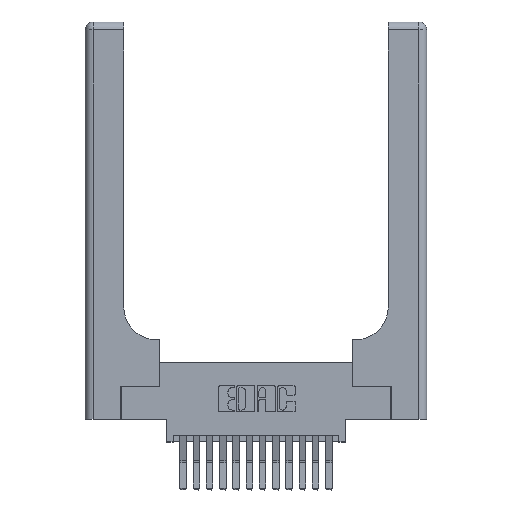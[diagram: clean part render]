
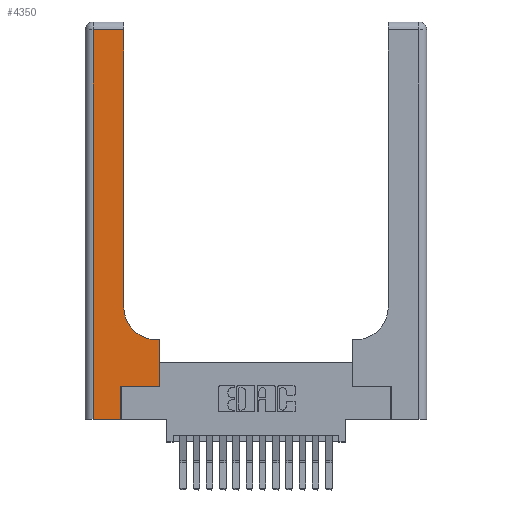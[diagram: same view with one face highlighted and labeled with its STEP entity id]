
A CAD part, top view. The second image highlights one B-rep face of the part: STEP entity #4350.
In plain terms, the highlighted planar face has unit normal (0, 0, 1).
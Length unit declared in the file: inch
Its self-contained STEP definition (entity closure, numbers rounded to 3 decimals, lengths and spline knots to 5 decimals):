
#340 = VERTEX_POINT ( 'NONE', #6474 ) ;
#570 = DIRECTION ( 'NONE',  ( 0., 1., 0. ) ) ;
#598 = CARTESIAN_POINT ( 'NONE',  ( 0.06, 3., 0.37 ) ) ;
#659 = DIRECTION ( 'NONE',  ( 0., 0., -1. ) ) ;
#872 = EDGE_CURVE ( 'NONE', #340, #6453, #12207, .T. ) ;
#1150 = CARTESIAN_POINT ( 'NONE',  ( 0.2915, 2.94, 0.37 ) ) ;
#1258 = VECTOR ( 'NONE', #15125, 39.37008 ) ;
#1740 = VECTOR ( 'NONE', #7307, 39.37008 ) ;
#1985 = DIRECTION ( 'NONE',  ( -1., 0., 0. ) ) ;
#2707 = FACE_OUTER_BOUND ( 'NONE', #17786, .T. ) ;
#3365 = PLANE ( 'NONE',  #12543 ) ;
#3429 = ORIENTED_EDGE ( 'NONE', *, *, #18812, .T. ) ;
#3630 = EDGE_CURVE ( 'NONE', #17448, #7913, #17579, .T. ) ;
#3677 = EDGE_CURVE ( 'NONE', #14177, #4645, #4109, .T. ) ;
#4024 = ORIENTED_EDGE ( 'NONE', *, *, #6787, .T. ) ;
#4109 = LINE ( 'NONE', #10282, #16007 ) ;
#4350 = ADVANCED_FACE ( 'NONE', ( #2707 ), #3365, .F. ) ;
#4645 = VERTEX_POINT ( 'NONE', #1150 ) ;
#4694 = EDGE_CURVE ( 'NONE', #4645, #11774, #6100, .T. ) ;
#4788 = ORIENTED_EDGE ( 'NONE', *, *, #872, .T. ) ;
#4884 = CIRCLE ( 'NONE', #17554, 0.25 ) ;
#5657 = CARTESIAN_POINT ( 'NONE',  ( 0.5585, 0.25, 0.37 ) ) ;
#5675 = DIRECTION ( 'NONE',  ( 1., 0., 0. ) ) ;
#5801 = VERTEX_POINT ( 'NONE', #12511 ) ;
#6100 = LINE ( 'NONE', #12879, #18028 ) ;
#6333 = VECTOR ( 'NONE', #10007, 39.37008 ) ;
#6453 = VERTEX_POINT ( 'NONE', #8918 ) ;
#6474 = CARTESIAN_POINT ( 'NONE',  ( 0.06, 0., 0.37 ) ) ;
#6666 = DIRECTION ( 'NONE',  ( 0., -1., 0. ) ) ;
#6787 = EDGE_CURVE ( 'NONE', #5801, #14177, #4884, .T. ) ;
#6846 = VECTOR ( 'NONE', #5675, 39.37008 ) ;
#7212 = CARTESIAN_POINT ( 'NONE',  ( 0.5585, 0.25, 0.37 ) ) ;
#7307 = DIRECTION ( 'NONE',  ( -1., 0., 0. ) ) ;
#7318 = EDGE_CURVE ( 'NONE', #6453, #17448, #17228, .T. ) ;
#7367 = ORIENTED_EDGE ( 'NONE', *, *, #10630, .T. ) ;
#7376 = CARTESIAN_POINT ( 'NONE',  ( 0.2915, 0.6, 0.37 ) ) ;
#7913 = VERTEX_POINT ( 'NONE', #7212 ) ;
#8918 = CARTESIAN_POINT ( 'NONE',  ( 0.269, 0., 0.37 ) ) ;
#9298 = CARTESIAN_POINT ( 'NONE',  ( 0., 0., 0.37 ) ) ;
#9314 = CARTESIAN_POINT ( 'NONE',  ( 0.5415, 0.85, 0.37 ) ) ;
#9747 = DIRECTION ( 'NONE',  ( -1., 0., 0. ) ) ;
#9983 = ORIENTED_EDGE ( 'NONE', *, *, #4694, .T. ) ;
#10007 = DIRECTION ( 'NONE',  ( 0., 1., 0. ) ) ;
#10282 = CARTESIAN_POINT ( 'NONE',  ( 0.2915, 3., 0.37 ) ) ;
#10399 = ORIENTED_EDGE ( 'NONE', *, *, #3630, .T. ) ;
#10630 = EDGE_CURVE ( 'NONE', #7913, #18612, #11393, .T. ) ;
#11393 = LINE ( 'NONE', #5657, #6333 ) ;
#11774 = VERTEX_POINT ( 'NONE', #15632 ) ;
#11779 = VECTOR ( 'NONE', #12365, 39.37008 ) ;
#11892 = CARTESIAN_POINT ( 'NONE',  ( 0.5585, 0.6, 0.37 ) ) ;
#11990 = ORIENTED_EDGE ( 'NONE', *, *, #7318, .T. ) ;
#12207 = LINE ( 'NONE', #9298, #1258 ) ;
#12365 = DIRECTION ( 'NONE',  ( 0., 1., 0. ) ) ;
#12457 = LINE ( 'NONE', #7376, #1740 ) ;
#12511 = CARTESIAN_POINT ( 'NONE',  ( 0.5415, 0.6, 0.37 ) ) ;
#12543 = AXIS2_PLACEMENT_3D ( 'NONE', #13532, #659, #1985 ) ;
#12879 = CARTESIAN_POINT ( 'NONE',  ( 0., 2.94, 0.37 ) ) ;
#13532 = CARTESIAN_POINT ( 'NONE',  ( 0., 3., 0.37 ) ) ;
#14177 = VERTEX_POINT ( 'NONE', #14612 ) ;
#14612 = CARTESIAN_POINT ( 'NONE',  ( 0.2915, 0.85, 0.37 ) ) ;
#14901 = CARTESIAN_POINT ( 'NONE',  ( 0.269, 0.25, 0.37 ) ) ;
#14933 = VECTOR ( 'NONE', #6666, 39.37008 ) ;
#15125 = DIRECTION ( 'NONE',  ( 1., 0., 0. ) ) ;
#15284 = CARTESIAN_POINT ( 'NONE',  ( 0.269, 0., 0.37 ) ) ;
#15632 = CARTESIAN_POINT ( 'NONE',  ( 0.06, 2.94, 0.37 ) ) ;
#15728 = CARTESIAN_POINT ( 'NONE',  ( 0.269, 0.25, 0.37 ) ) ;
#15819 = ORIENTED_EDGE ( 'NONE', *, *, #3677, .T. ) ;
#15828 = DIRECTION ( 'NONE',  ( 1., 0., 0. ) ) ;
#16005 = EDGE_CURVE ( 'NONE', #18612, #5801, #12457, .T. ) ;
#16007 = VECTOR ( 'NONE', #570, 39.37008 ) ;
#16098 = LINE ( 'NONE', #598, #14933 ) ;
#16337 = ORIENTED_EDGE ( 'NONE', *, *, #16005, .T. ) ;
#17228 = LINE ( 'NONE', #15284, #11779 ) ;
#17448 = VERTEX_POINT ( 'NONE', #14901 ) ;
#17554 = AXIS2_PLACEMENT_3D ( 'NONE', #9314, #18530, #15828 ) ;
#17579 = LINE ( 'NONE', #15728, #6846 ) ;
#17786 = EDGE_LOOP ( 'NONE', ( #15819, #9983, #3429, #4788, #11990, #10399, #7367, #16337, #4024 ) ) ;
#18028 = VECTOR ( 'NONE', #9747, 39.37008 ) ;
#18530 = DIRECTION ( 'NONE',  ( 0., 0., -1. ) ) ;
#18612 = VERTEX_POINT ( 'NONE', #11892 ) ;
#18812 = EDGE_CURVE ( 'NONE', #11774, #340, #16098, .T. ) ;
